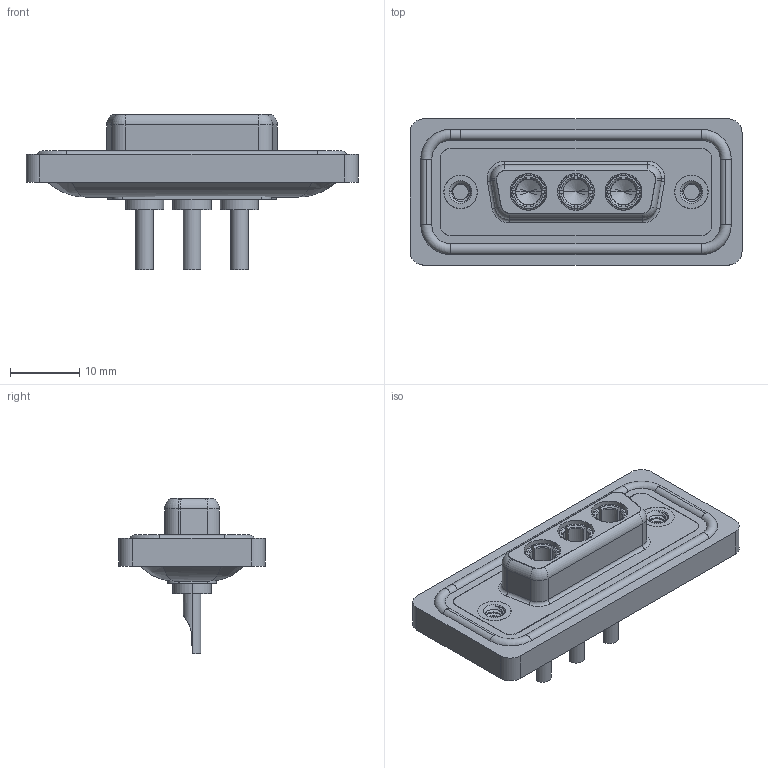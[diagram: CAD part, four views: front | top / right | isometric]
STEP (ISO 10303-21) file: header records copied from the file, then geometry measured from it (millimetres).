
FILE_DESCRIPTION (( 'STEP AP203' ), '1' );
FILE_NAME ('628W3W3-222-1N2.STEP', '2024-03-22T14:16:28', ( '' ), ( '' ), 'SwSTEP 2.0', 'SolidWorks 2023', '' );
FILE_SCHEMA (( 'CONFIG_CONTROL_DESIGN' ));
Length unit declared in the file: millimetre
Products named in the file (7): 628Combo Waterproof Housing_15 Contacts; Power Socket_10A SC; 628W3W3-222-1N2; 628Combo Threaded Rivet_2; 628Combo Shell Front_15 Contacts; 628Combo Shell Rear_15 Contacts; 628Combo Housing_3W3
Assembly tree (9 placements, depth 2):
  628W3W3-222-1N2
    628Combo Housing_3W3
    628Combo Waterproof Housing_15 Contacts
    628Combo Shell Front_15 Contacts
    628Combo Shell Rear_15 Contacts
    628Combo Threaded Rivet_2  x2
    Power Socket_10A SC  x3
Bounding box: 47.9 x 21.1 x 22.45 mm (x, y, z)
Volume: 6018.1 mm3; surface area: 9881.7 mm2
Topology: 13 solids, 13 shells, 623 faces, 1587 edges, 1000 vertices
Faces by surface type: cylinder 266, plane 198, torus 83, cone 63, bspline 13
Entity records: 16036 total; most frequent: CARTESIAN_POINT 4534, DIRECTION 2346, ORIENTED_EDGE 2200, EDGE_CURVE 1100, AXIS2_PLACEMENT_3D 935, VERTEX_POINT 696, CIRCLE 489, EDGE_LOOP 486
